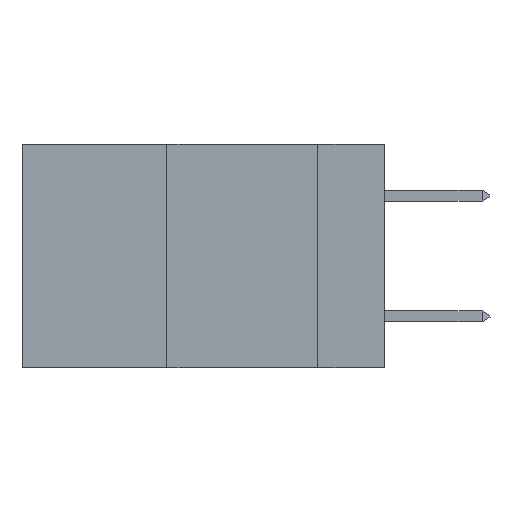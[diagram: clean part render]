
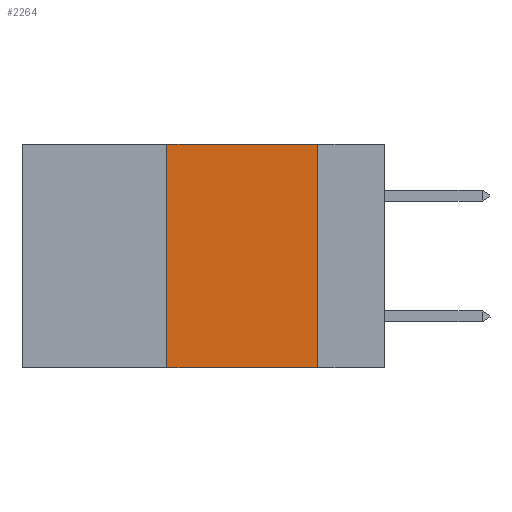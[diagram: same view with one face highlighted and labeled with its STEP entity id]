
A CAD part, left-side view. The second image highlights one B-rep face of the part: STEP entity #2264.
In plain terms, the highlighted planar face has unit normal (-1, 0, 0).
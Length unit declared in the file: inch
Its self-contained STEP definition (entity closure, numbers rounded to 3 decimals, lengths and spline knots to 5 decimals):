
#79 = VECTOR ( 'NONE', #6760, 39.37008 ) ;
#208 = DIRECTION ( 'NONE',  ( 0., 0., -1. ) ) ;
#277 = DIRECTION ( 'NONE',  ( 1., 0., 0. ) ) ;
#451 = ORIENTED_EDGE ( 'NONE', *, *, #500, .F. ) ;
#475 = ORIENTED_EDGE ( 'NONE', *, *, #6074, .F. ) ;
#500 = EDGE_CURVE ( 'NONE', #3264, #1853, #829, .T. ) ;
#829 = LINE ( 'NONE', #1825, #8706 ) ;
#980 = EDGE_CURVE ( 'NONE', #3481, #6838, #2212, .T. ) ;
#1516 = CARTESIAN_POINT ( 'NONE',  ( 0., 0.6, -0.37 ) ) ;
#1825 = CARTESIAN_POINT ( 'NONE',  ( 0., 0.11, 0. ) ) ;
#1853 = VERTEX_POINT ( 'NONE', #4200 ) ;
#2017 = DIRECTION ( 'NONE',  ( 0., -1., 0. ) ) ;
#2212 = LINE ( 'NONE', #8360, #79 ) ;
#2264 = ADVANCED_FACE ( 'NONE', ( #5358 ), #5022, .F. ) ;
#2308 = LINE ( 'NONE', #1516, #8546 ) ;
#2880 = CARTESIAN_POINT ( 'NONE',  ( 0., 0.36, 0. ) ) ;
#3264 = VERTEX_POINT ( 'NONE', #4906 ) ;
#3444 = EDGE_LOOP ( 'NONE', ( #451, #475, #7521, #5472 ) ) ;
#3481 = VERTEX_POINT ( 'NONE', #6171 ) ;
#3847 = LINE ( 'NONE', #6031, #10045 ) ;
#4200 = CARTESIAN_POINT ( 'NONE',  ( 0., 0.11, -0.37 ) ) ;
#4906 = CARTESIAN_POINT ( 'NONE',  ( 0., 0.11, 0. ) ) ;
#5022 = PLANE ( 'NONE',  #5737 ) ;
#5130 = DIRECTION ( 'NONE',  ( 0., 0., -1. ) ) ;
#5358 = FACE_OUTER_BOUND ( 'NONE', #3444, .T. ) ;
#5391 = EDGE_CURVE ( 'NONE', #3481, #1853, #2308, .T. ) ;
#5472 = ORIENTED_EDGE ( 'NONE', *, *, #5391, .T. ) ;
#5737 = AXIS2_PLACEMENT_3D ( 'NONE', #7482, #277, #208 ) ;
#6031 = CARTESIAN_POINT ( 'NONE',  ( 0., 0.6, 0. ) ) ;
#6074 = EDGE_CURVE ( 'NONE', #6838, #3264, #3847, .T. ) ;
#6171 = CARTESIAN_POINT ( 'NONE',  ( 0., 0.36, -0.37 ) ) ;
#6311 = DIRECTION ( 'NONE',  ( 0., -1., 0. ) ) ;
#6760 = DIRECTION ( 'NONE',  ( 0., 0., 1. ) ) ;
#6838 = VERTEX_POINT ( 'NONE', #2880 ) ;
#7482 = CARTESIAN_POINT ( 'NONE',  ( 0., 0.6, 0. ) ) ;
#7521 = ORIENTED_EDGE ( 'NONE', *, *, #980, .F. ) ;
#8360 = CARTESIAN_POINT ( 'NONE',  ( 0., 0.36, 0. ) ) ;
#8546 = VECTOR ( 'NONE', #6311, 39.37008 ) ;
#8706 = VECTOR ( 'NONE', #5130, 39.37008 ) ;
#10045 = VECTOR ( 'NONE', #2017, 39.37008 ) ;
